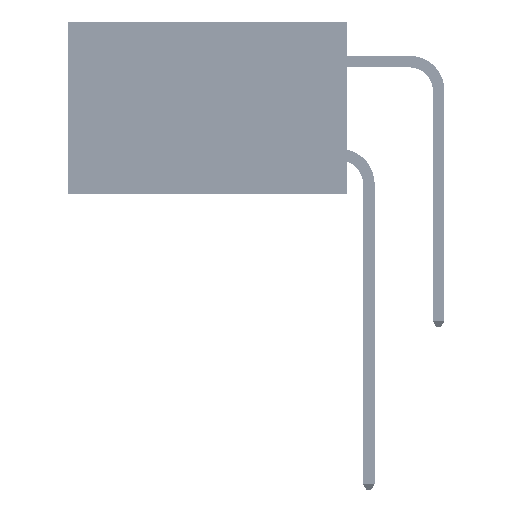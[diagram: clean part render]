
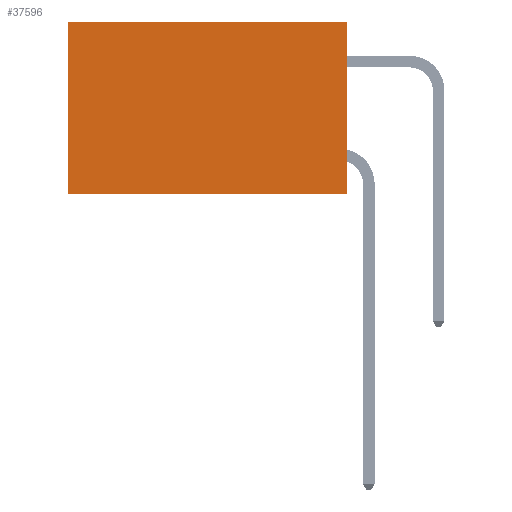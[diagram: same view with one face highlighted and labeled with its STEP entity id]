
A CAD part, left-side view. The second image highlights one B-rep face of the part: STEP entity #37596.
In plain terms, the highlighted planar face has unit normal (-1, 0, 0).
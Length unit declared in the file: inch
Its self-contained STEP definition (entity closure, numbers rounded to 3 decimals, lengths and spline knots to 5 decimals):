
#305 = ORIENTED_EDGE ( 'NONE', *, *, #22794, .T. ) ;
#393 = PLANE ( 'NONE',  #4861 ) ;
#726 = CARTESIAN_POINT ( 'NONE',  ( 0.2875, 0., 0. ) ) ;
#1460 = CARTESIAN_POINT ( 'NONE',  ( 0.2875, 0.6, 0. ) ) ;
#2340 = DIRECTION ( 'NONE',  ( 0., 0., -1. ) ) ;
#3719 = VERTEX_POINT ( 'NONE', #46431 ) ;
#4861 = AXIS2_PLACEMENT_3D ( 'NONE', #726, #30091, #41764 ) ;
#5035 = DIRECTION ( 'NONE',  ( 0., 0., -1. ) ) ;
#5386 = VECTOR ( 'NONE', #2340, 39.37008 ) ;
#6729 = CARTESIAN_POINT ( 'NONE',  ( 0.2875, 0.6, 0. ) ) ;
#11459 = DIRECTION ( 'NONE',  ( 0., 1., 0. ) ) ;
#12952 = DIRECTION ( 'NONE',  ( 0., 1., 0. ) ) ;
#15218 = VECTOR ( 'NONE', #11459, 39.37008 ) ;
#15693 = EDGE_CURVE ( 'NONE', #19131, #3719, #25227, .T. ) ;
#16233 = VERTEX_POINT ( 'NONE', #44385 ) ;
#18682 = VECTOR ( 'NONE', #5035, 39.37008 ) ;
#19131 = VERTEX_POINT ( 'NONE', #27678 ) ;
#22622 = LINE ( 'NONE', #1460, #18682 ) ;
#22794 = EDGE_CURVE ( 'NONE', #16233, #46494, #36232, .T. ) ;
#22876 = ORIENTED_EDGE ( 'NONE', *, *, #15693, .F. ) ;
#25227 = LINE ( 'NONE', #30400, #15218 ) ;
#25277 = CARTESIAN_POINT ( 'NONE',  ( 0.2875, 0., 0. ) ) ;
#25913 = LINE ( 'NONE', #25277, #5386 ) ;
#27678 = CARTESIAN_POINT ( 'NONE',  ( 0.2875, 0., -0.37 ) ) ;
#28600 = VECTOR ( 'NONE', #12952, 39.37008 ) ;
#28880 = EDGE_CURVE ( 'NONE', #16233, #19131, #25913, .T. ) ;
#30091 = DIRECTION ( 'NONE',  ( 1., 0., 0. ) ) ;
#30400 = CARTESIAN_POINT ( 'NONE',  ( 0.2875, 0., -0.37 ) ) ;
#30930 = ORIENTED_EDGE ( 'NONE', *, *, #28880, .F. ) ;
#36232 = LINE ( 'NONE', #42925, #28600 ) ;
#37596 = ADVANCED_FACE ( 'NONE', ( #46176 ), #393, .F. ) ;
#41009 = EDGE_LOOP ( 'NONE', ( #48385, #22876, #30930, #305 ) ) ;
#41764 = DIRECTION ( 'NONE',  ( 0., 0., -1. ) ) ;
#42072 = EDGE_CURVE ( 'NONE', #46494, #3719, #22622, .T. ) ;
#42925 = CARTESIAN_POINT ( 'NONE',  ( 0.2875, 0., 0. ) ) ;
#44385 = CARTESIAN_POINT ( 'NONE',  ( 0.2875, 0., 0. ) ) ;
#46176 = FACE_OUTER_BOUND ( 'NONE', #41009, .T. ) ;
#46431 = CARTESIAN_POINT ( 'NONE',  ( 0.2875, 0.6, -0.37 ) ) ;
#46494 = VERTEX_POINT ( 'NONE', #6729 ) ;
#48385 = ORIENTED_EDGE ( 'NONE', *, *, #42072, .T. ) ;
